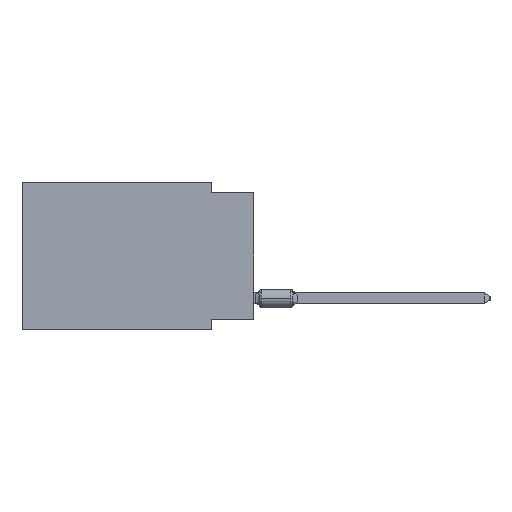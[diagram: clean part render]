
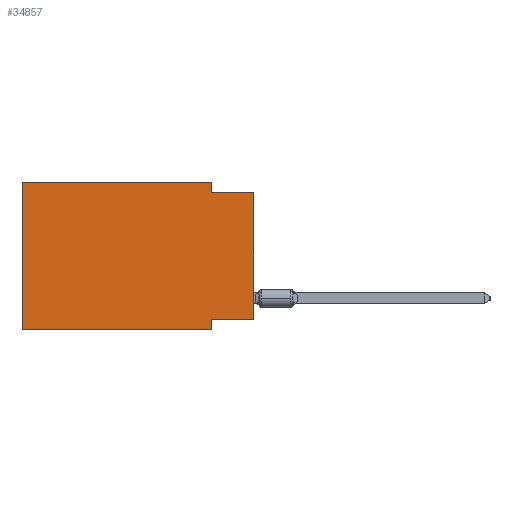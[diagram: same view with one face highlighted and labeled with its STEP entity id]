
A CAD part, left-side view. The second image highlights one B-rep face of the part: STEP entity #34857.
In plain terms, the highlighted planar face has unit normal (-1, 0, 0).
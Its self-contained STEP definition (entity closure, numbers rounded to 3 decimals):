
#1915 = LINE ( 'NONE', #26668, #51337 ) ;
#2645 = DIRECTION ( 'NONE',  ( 0., 0., 1. ) ) ;
#3268 = LINE ( 'NONE', #91213, #15957 ) ;
#6441 = DIRECTION ( 'NONE',  ( 0., 1., 0. ) ) ;
#6663 = CARTESIAN_POINT ( 'NONE',  ( 0., 0., -0.635 ) ) ;
#14066 = LINE ( 'NONE', #6663, #45560 ) ;
#14092 = ORIENTED_EDGE ( 'NONE', *, *, #99633, .F. ) ;
#15957 = VECTOR ( 'NONE', #36425, 1000. ) ;
#20703 = LINE ( 'NONE', #101252, #102879 ) ;
#21286 = EDGE_CURVE ( 'NONE', #101187, #67427, #1915, .T. ) ;
#21634 = DIRECTION ( 'NONE',  ( 1., 0., 0. ) ) ;
#22724 = EDGE_CURVE ( 'NONE', #81002, #27307, #102440, .T. ) ;
#23722 = CARTESIAN_POINT ( 'NONE',  ( 0., 13.97, 0. ) ) ;
#25786 = PLANE ( 'NONE',  #89353 ) ;
#26038 = ORIENTED_EDGE ( 'NONE', *, *, #21286, .F. ) ;
#26668 = CARTESIAN_POINT ( 'NONE',  ( 0., 2.54, 0. ) ) ;
#27042 = EDGE_CURVE ( 'NONE', #81002, #29881, #3268, .T. ) ;
#27307 = VERTEX_POINT ( 'NONE', #23722 ) ;
#28699 = EDGE_CURVE ( 'NONE', #56817, #69851, #43200, .T. ) ;
#29881 = VERTEX_POINT ( 'NONE', #53616 ) ;
#31653 = ORIENTED_EDGE ( 'NONE', *, *, #68526, .F. ) ;
#33402 = VECTOR ( 'NONE', #98362, 1000. ) ;
#33572 = CARTESIAN_POINT ( 'NONE',  ( 0., 2.54, 0. ) ) ;
#34857 = ADVANCED_FACE ( 'NONE', ( #88436 ), #25786, .F. ) ;
#35919 = VECTOR ( 'NONE', #102234, 1000. ) ;
#36425 = DIRECTION ( 'NONE',  ( 0., -1., 0. ) ) ;
#36954 = CARTESIAN_POINT ( 'NONE',  ( 0., 13.97, -8.89 ) ) ;
#37387 = ORIENTED_EDGE ( 'NONE', *, *, #70671, .F. ) ;
#43200 = LINE ( 'NONE', #74795, #64977 ) ;
#43459 = EDGE_CURVE ( 'NONE', #56817, #92918, #20703, .T. ) ;
#45560 = VECTOR ( 'NONE', #46185, 1000. ) ;
#46185 = DIRECTION ( 'NONE',  ( 0., -1., 0. ) ) ;
#46862 = CARTESIAN_POINT ( 'NONE',  ( 0., 2.54, -8.255 ) ) ;
#51337 = VECTOR ( 'NONE', #75608, 1000. ) ;
#53616 = CARTESIAN_POINT ( 'NONE',  ( 0., 2.54, -8.89 ) ) ;
#54210 = EDGE_LOOP ( 'NONE', ( #89467, #37387, #26038, #31653, #82686, #88273, #14092, #62876 ) ) ;
#56817 = VERTEX_POINT ( 'NONE', #72777 ) ;
#58256 = VECTOR ( 'NONE', #86604, 1000. ) ;
#62408 = CARTESIAN_POINT ( 'NONE',  ( 0., 13.97, 0. ) ) ;
#62876 = ORIENTED_EDGE ( 'NONE', *, *, #43459, .F. ) ;
#64977 = VECTOR ( 'NONE', #2645, 1000. ) ;
#67427 = VERTEX_POINT ( 'NONE', #67786 ) ;
#67786 = CARTESIAN_POINT ( 'NONE',  ( 0., 2.54, -0.635 ) ) ;
#68526 = EDGE_CURVE ( 'NONE', #27307, #101187, #75675, .T. ) ;
#69851 = VERTEX_POINT ( 'NONE', #87191 ) ;
#70105 = CARTESIAN_POINT ( 'NONE',  ( 0., 2.54, -8.89 ) ) ;
#70671 = EDGE_CURVE ( 'NONE', #67427, #69851, #14066, .T. ) ;
#72777 = CARTESIAN_POINT ( 'NONE',  ( 0., 0., -8.255 ) ) ;
#74127 = CARTESIAN_POINT ( 'NONE',  ( 0., 13.97, 0. ) ) ;
#74795 = CARTESIAN_POINT ( 'NONE',  ( 0., 0., 0. ) ) ;
#75608 = DIRECTION ( 'NONE',  ( 0., 0., -1. ) ) ;
#75675 = LINE ( 'NONE', #74127, #33402 ) ;
#81002 = VERTEX_POINT ( 'NONE', #36954 ) ;
#82686 = ORIENTED_EDGE ( 'NONE', *, *, #22724, .F. ) ;
#86604 = DIRECTION ( 'NONE',  ( 0., 0., 1. ) ) ;
#87191 = CARTESIAN_POINT ( 'NONE',  ( 0., 0., -0.635 ) ) ;
#88273 = ORIENTED_EDGE ( 'NONE', *, *, #27042, .T. ) ;
#88436 = FACE_OUTER_BOUND ( 'NONE', #54210, .T. ) ;
#89353 = AXIS2_PLACEMENT_3D ( 'NONE', #96351, #21634, #102706 ) ;
#89467 = ORIENTED_EDGE ( 'NONE', *, *, #28699, .T. ) ;
#91213 = CARTESIAN_POINT ( 'NONE',  ( 0., 13.97, -8.89 ) ) ;
#92918 = VERTEX_POINT ( 'NONE', #46862 ) ;
#96351 = CARTESIAN_POINT ( 'NONE',  ( 0., 13.97, 0. ) ) ;
#98362 = DIRECTION ( 'NONE',  ( 0., -1., 0. ) ) ;
#99633 = EDGE_CURVE ( 'NONE', #92918, #29881, #103265, .T. ) ;
#101187 = VERTEX_POINT ( 'NONE', #33572 ) ;
#101252 = CARTESIAN_POINT ( 'NONE',  ( 0., 0., -8.255 ) ) ;
#102234 = DIRECTION ( 'NONE',  ( 0., 0., -1. ) ) ;
#102440 = LINE ( 'NONE', #62408, #58256 ) ;
#102706 = DIRECTION ( 'NONE',  ( 0., 0., -1. ) ) ;
#102879 = VECTOR ( 'NONE', #6441, 1000. ) ;
#103265 = LINE ( 'NONE', #70105, #35919 ) ;
